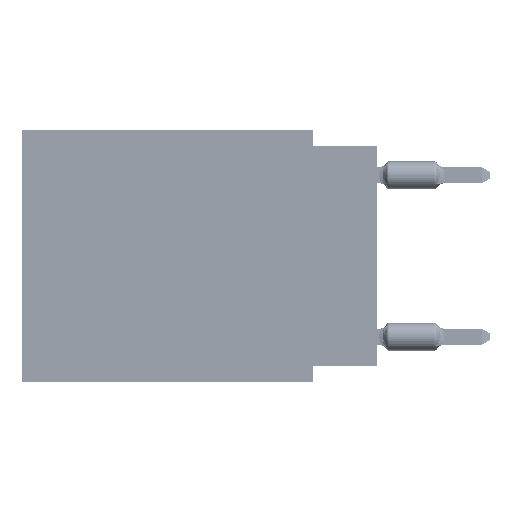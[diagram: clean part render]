
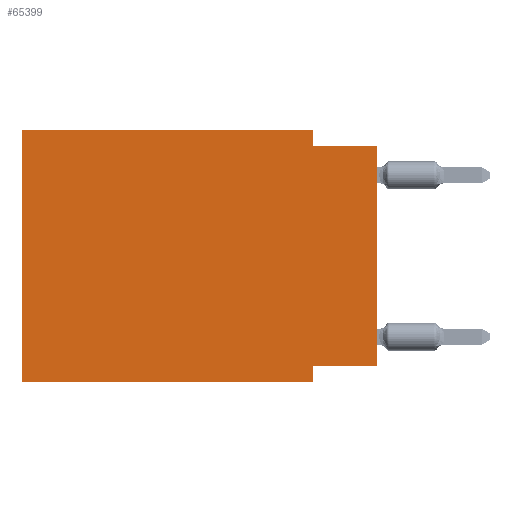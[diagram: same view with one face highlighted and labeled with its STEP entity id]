
A CAD part, left-side view. The second image highlights one B-rep face of the part: STEP entity #65399.
In plain terms, the highlighted planar face has unit normal (-1, 0, 0).
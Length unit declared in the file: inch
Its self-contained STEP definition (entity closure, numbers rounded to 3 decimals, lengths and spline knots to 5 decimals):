
#1028 = ORIENTED_EDGE ( 'NONE', *, *, #1337, .T. ) ;
#1337 = EDGE_CURVE ( 'NONE', #29646, #64374, #10080, .T. ) ;
#1659 = VECTOR ( 'NONE', #23194, 39.37008 ) ;
#1852 = CARTESIAN_POINT ( 'NONE',  ( 0., 0., -0.025 ) ) ;
#3565 = DIRECTION ( 'NONE',  ( 0., -1., 0. ) ) ;
#5730 = LINE ( 'NONE', #17702, #16906 ) ;
#7948 = VECTOR ( 'NONE', #34293, 39.37008 ) ;
#8970 = LINE ( 'NONE', #62459, #76730 ) ;
#10080 = LINE ( 'NONE', #58739, #1659 ) ;
#10739 = CARTESIAN_POINT ( 'NONE',  ( 0., 0., -0.025 ) ) ;
#11631 = VECTOR ( 'NONE', #27251, 39.37008 ) ;
#12691 = EDGE_LOOP ( 'NONE', ( #1028, #38153, #63961, #46966, #36176, #53336, #30776, #40337 ) ) ;
#12899 = VERTEX_POINT ( 'NONE', #27295 ) ;
#15431 = VERTEX_POINT ( 'NONE', #68845 ) ;
#16858 = PLANE ( 'NONE',  #71899 ) ;
#16906 = VECTOR ( 'NONE', #18483, 39.37008 ) ;
#16913 = EDGE_CURVE ( 'NONE', #27764, #47415, #8970, .T. ) ;
#17265 = EDGE_CURVE ( 'NONE', #31408, #12899, #76196, .T. ) ;
#17702 = CARTESIAN_POINT ( 'NONE',  ( 0., 0.55, -0.39 ) ) ;
#17913 = CARTESIAN_POINT ( 'NONE',  ( 0., 0.55, 0. ) ) ;
#18483 = DIRECTION ( 'NONE',  ( 0., -1., 0. ) ) ;
#20508 = LINE ( 'NONE', #44861, #11631 ) ;
#22042 = CARTESIAN_POINT ( 'NONE',  ( 0., 0.55, 0. ) ) ;
#23194 = DIRECTION ( 'NONE',  ( 0., 0., 1. ) ) ;
#27251 = DIRECTION ( 'NONE',  ( 0., 1., 0. ) ) ;
#27295 = CARTESIAN_POINT ( 'NONE',  ( 0., 0.1, -0.025 ) ) ;
#27764 = VERTEX_POINT ( 'NONE', #77022 ) ;
#28723 = CARTESIAN_POINT ( 'NONE',  ( 0., 0.1, 0. ) ) ;
#29646 = VERTEX_POINT ( 'NONE', #57711 ) ;
#30463 = VECTOR ( 'NONE', #40696, 39.37008 ) ;
#30776 = ORIENTED_EDGE ( 'NONE', *, *, #16913, .F. ) ;
#31408 = VERTEX_POINT ( 'NONE', #28723 ) ;
#32506 = EDGE_CURVE ( 'NONE', #29646, #27764, #20508, .T. ) ;
#33902 = EDGE_CURVE ( 'NONE', #61069, #47415, #5730, .T. ) ;
#34293 = DIRECTION ( 'NONE',  ( 0., 0., -1. ) ) ;
#35218 = DIRECTION ( 'NONE',  ( 0., 0., -1. ) ) ;
#35871 = LINE ( 'NONE', #17913, #30463 ) ;
#36176 = ORIENTED_EDGE ( 'NONE', *, *, #57060, .F. ) ;
#38153 = ORIENTED_EDGE ( 'NONE', *, *, #77211, .F. ) ;
#40337 = ORIENTED_EDGE ( 'NONE', *, *, #32506, .F. ) ;
#40696 = DIRECTION ( 'NONE',  ( 0., -1., 0. ) ) ;
#40822 = DIRECTION ( 'NONE',  ( 1., 0., 0. ) ) ;
#42570 = LINE ( 'NONE', #49353, #78585 ) ;
#42957 = DIRECTION ( 'NONE',  ( 0., 0., 1. ) ) ;
#44861 = CARTESIAN_POINT ( 'NONE',  ( 0., 0., -0.365 ) ) ;
#46966 = ORIENTED_EDGE ( 'NONE', *, *, #73333, .F. ) ;
#47191 = CARTESIAN_POINT ( 'NONE',  ( 0., 0.55, -0.39 ) ) ;
#47415 = VERTEX_POINT ( 'NONE', #58574 ) ;
#49353 = CARTESIAN_POINT ( 'NONE',  ( 0., 0.55, 0. ) ) ;
#51633 = VECTOR ( 'NONE', #3565, 39.37008 ) ;
#53336 = ORIENTED_EDGE ( 'NONE', *, *, #33902, .T. ) ;
#57060 = EDGE_CURVE ( 'NONE', #61069, #15431, #42570, .T. ) ;
#57711 = CARTESIAN_POINT ( 'NONE',  ( 0., 0., -0.365 ) ) ;
#58574 = CARTESIAN_POINT ( 'NONE',  ( 0., 0.1, -0.39 ) ) ;
#58739 = CARTESIAN_POINT ( 'NONE',  ( 0., 0., 0. ) ) ;
#61069 = VERTEX_POINT ( 'NONE', #47191 ) ;
#62459 = CARTESIAN_POINT ( 'NONE',  ( 0., 0.1, -0.39 ) ) ;
#62840 = DIRECTION ( 'NONE',  ( 0., 0., -1. ) ) ;
#63961 = ORIENTED_EDGE ( 'NONE', *, *, #17265, .F. ) ;
#64205 = CARTESIAN_POINT ( 'NONE',  ( 0., 0.1, 0. ) ) ;
#64374 = VERTEX_POINT ( 'NONE', #1852 ) ;
#65378 = LINE ( 'NONE', #10739, #51633 ) ;
#65399 = ADVANCED_FACE ( 'NONE', ( #77109 ), #16858, .F. ) ;
#68845 = CARTESIAN_POINT ( 'NONE',  ( 0., 0.55, 0. ) ) ;
#71899 = AXIS2_PLACEMENT_3D ( 'NONE', #22042, #40822, #35218 ) ;
#73333 = EDGE_CURVE ( 'NONE', #15431, #31408, #35871, .T. ) ;
#76196 = LINE ( 'NONE', #64205, #7948 ) ;
#76730 = VECTOR ( 'NONE', #62840, 39.37008 ) ;
#77022 = CARTESIAN_POINT ( 'NONE',  ( 0., 0.1, -0.365 ) ) ;
#77109 = FACE_OUTER_BOUND ( 'NONE', #12691, .T. ) ;
#77211 = EDGE_CURVE ( 'NONE', #12899, #64374, #65378, .T. ) ;
#78585 = VECTOR ( 'NONE', #42957, 39.37008 ) ;
